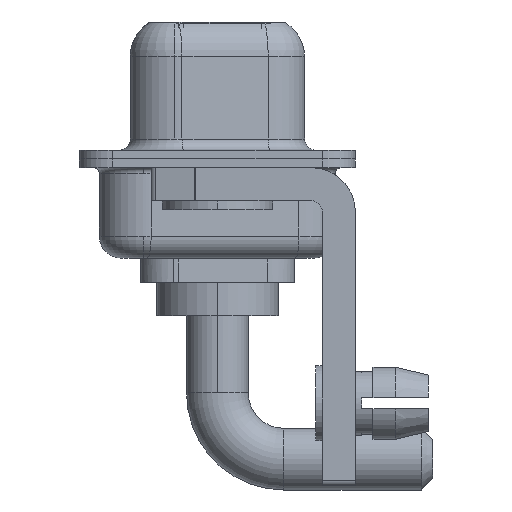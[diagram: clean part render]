
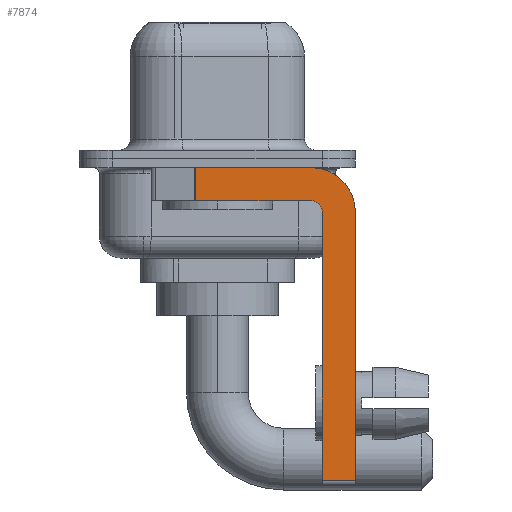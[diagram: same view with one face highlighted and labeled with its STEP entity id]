
A CAD part, left-side view. The second image highlights one B-rep face of the part: STEP entity #7874.
In plain terms, the highlighted planar face has unit normal (-1, 0, 0).
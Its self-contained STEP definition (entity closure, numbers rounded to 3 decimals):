
#354 = VERTEX_POINT ( 'NONE', #9096 ) ;
#741 = VECTOR ( 'NONE', #10701, 1000. ) ;
#774 = CARTESIAN_POINT ( 'NONE',  ( -2.9, -6.25, -14.55 ) ) ;
#894 = PLANE ( 'NONE',  #13384 ) ;
#1049 = VERTEX_POINT ( 'NONE', #11549 ) ;
#1103 = VECTOR ( 'NONE', #1777, 1000. ) ;
#1635 = VERTEX_POINT ( 'NONE', #2751 ) ;
#1777 = DIRECTION ( 'NONE',  ( 0., 1., 0. ) ) ;
#2195 = DIRECTION ( 'NONE',  ( 0., -1., 0. ) ) ;
#2548 = DIRECTION ( 'NONE',  ( 0., -1., 0. ) ) ;
#2751 = CARTESIAN_POINT ( 'NONE',  ( -2.9, 0.978, -1.9 ) ) ;
#3116 = EDGE_CURVE ( 'NONE', #13886, #1049, #12739, .T. ) ;
#3353 = DIRECTION ( 'NONE',  ( 0., 0., -1. ) ) ;
#3376 = ORIENTED_EDGE ( 'NONE', *, *, #10709, .F. ) ;
#3474 = CARTESIAN_POINT ( 'NONE',  ( -2.9, -4.75, -14.55 ) ) ;
#3491 = CARTESIAN_POINT ( 'NONE',  ( -2.9, -4.25, -2.4 ) ) ;
#3943 = VECTOR ( 'NONE', #2195, 1000. ) ;
#4348 = VERTEX_POINT ( 'NONE', #774 ) ;
#4392 = CARTESIAN_POINT ( 'NONE',  ( -2.9, -4.25, -1.9 ) ) ;
#4665 = LINE ( 'NONE', #13034, #3943 ) ;
#4879 = FACE_OUTER_BOUND ( 'NONE', #8506, .T. ) ;
#6309 = VERTEX_POINT ( 'NONE', #7984 ) ;
#6719 = LINE ( 'NONE', #4392, #1103 ) ;
#6727 = VECTOR ( 'NONE', #7062, 1000. ) ;
#6894 = DIRECTION ( 'NONE',  ( 0., 0., -1. ) ) ;
#6965 = EDGE_CURVE ( 'NONE', #8686, #4348, #11096, .T. ) ;
#7062 = DIRECTION ( 'NONE',  ( 0., 0., -1. ) ) ;
#7203 = ORIENTED_EDGE ( 'NONE', *, *, #7924, .F. ) ;
#7374 = VECTOR ( 'NONE', #2548, 1000. ) ;
#7500 = CARTESIAN_POINT ( 'NONE',  ( -2.9, -6.25, -2.4 ) ) ;
#7526 = CIRCLE ( 'NONE', #8508, 2. ) ;
#7822 = EDGE_CURVE ( 'NONE', #8686, #13886, #9524, .T. ) ;
#7860 = VECTOR ( 'NONE', #8674, 1000. ) ;
#7874 = ADVANCED_FACE ( 'NONE', ( #4879 ), #894, .F. ) ;
#7924 = EDGE_CURVE ( 'NONE', #354, #4348, #9854, .T. ) ;
#7984 = CARTESIAN_POINT ( 'NONE',  ( -2.9, 0.978, -0.4 ) ) ;
#8351 = DIRECTION ( 'NONE',  ( 0., 0., 1. ) ) ;
#8506 = EDGE_LOOP ( 'NONE', ( #3376, #12331, #8880, #14055, #14197, #12816, #7203, #15377 ) ) ;
#8508 = AXIS2_PLACEMENT_3D ( 'NONE', #13013, #9316, #6894 ) ;
#8674 = DIRECTION ( 'NONE',  ( 0., 0., -1. ) ) ;
#8686 = VERTEX_POINT ( 'NONE', #3474 ) ;
#8735 = CARTESIAN_POINT ( 'NONE',  ( -2.9, -4.25, -14.55 ) ) ;
#8880 = ORIENTED_EDGE ( 'NONE', *, *, #9523, .F. ) ;
#9096 = CARTESIAN_POINT ( 'NONE',  ( -2.9, -6.25, -2.4 ) ) ;
#9259 = EDGE_CURVE ( 'NONE', #6309, #1635, #11540, .T. ) ;
#9316 = DIRECTION ( 'NONE',  ( 1., 0., 0. ) ) ;
#9339 = CARTESIAN_POINT ( 'NONE',  ( -2.9, 0.978, -1.9 ) ) ;
#9451 = AXIS2_PLACEMENT_3D ( 'NONE', #3491, #9598, #8351 ) ;
#9523 = EDGE_CURVE ( 'NONE', #1049, #1635, #6719, .T. ) ;
#9524 = LINE ( 'NONE', #15632, #741 ) ;
#9598 = DIRECTION ( 'NONE',  ( -1., 0., 0. ) ) ;
#9854 = LINE ( 'NONE', #7500, #7860 ) ;
#10556 = CARTESIAN_POINT ( 'NONE',  ( -2.9, -4.25, -2.4 ) ) ;
#10690 = CARTESIAN_POINT ( 'NONE',  ( -2.9, -4.75, -2.4 ) ) ;
#10701 = DIRECTION ( 'NONE',  ( 0., 0., 1. ) ) ;
#10709 = EDGE_CURVE ( 'NONE', #6309, #12010, #4665, .T. ) ;
#11096 = LINE ( 'NONE', #8735, #7374 ) ;
#11326 = EDGE_CURVE ( 'NONE', #12010, #354, #7526, .T. ) ;
#11423 = CARTESIAN_POINT ( 'NONE',  ( -2.9, -4.25, -0.4 ) ) ;
#11540 = LINE ( 'NONE', #9339, #6727 ) ;
#11549 = CARTESIAN_POINT ( 'NONE',  ( -2.9, -4.25, -1.9 ) ) ;
#12010 = VERTEX_POINT ( 'NONE', #11423 ) ;
#12331 = ORIENTED_EDGE ( 'NONE', *, *, #9259, .T. ) ;
#12739 = CIRCLE ( 'NONE', #9451, 0.5 ) ;
#12816 = ORIENTED_EDGE ( 'NONE', *, *, #6965, .T. ) ;
#13013 = CARTESIAN_POINT ( 'NONE',  ( -2.9, -4.25, -2.4 ) ) ;
#13034 = CARTESIAN_POINT ( 'NONE',  ( -2.9, 3., -0.4 ) ) ;
#13384 = AXIS2_PLACEMENT_3D ( 'NONE', #10556, #15406, #3353 ) ;
#13886 = VERTEX_POINT ( 'NONE', #10690 ) ;
#14055 = ORIENTED_EDGE ( 'NONE', *, *, #3116, .F. ) ;
#14197 = ORIENTED_EDGE ( 'NONE', *, *, #7822, .F. ) ;
#15377 = ORIENTED_EDGE ( 'NONE', *, *, #11326, .F. ) ;
#15406 = DIRECTION ( 'NONE',  ( 1., 0., 0. ) ) ;
#15632 = CARTESIAN_POINT ( 'NONE',  ( -2.9, -4.75, -14.8 ) ) ;
